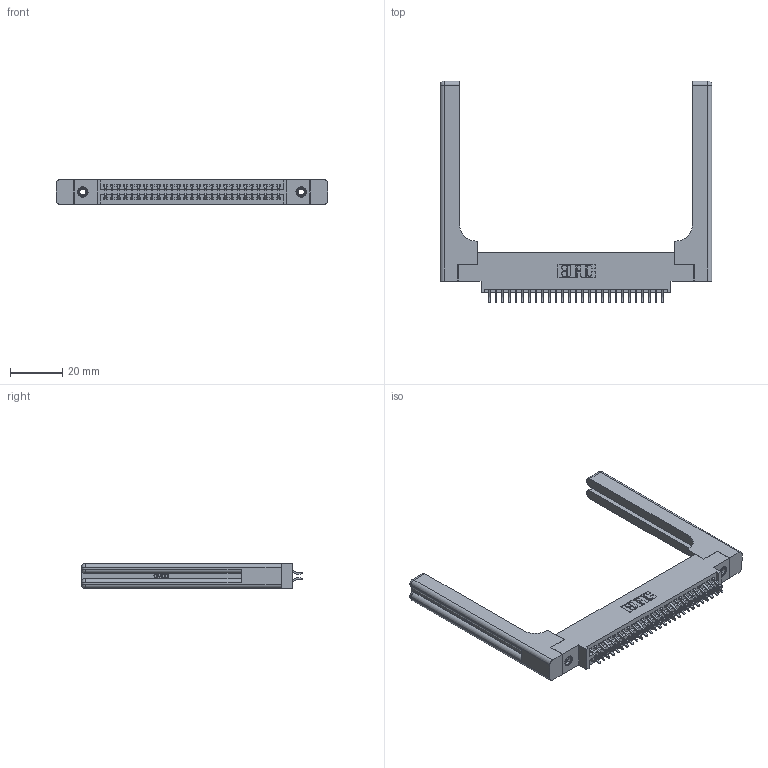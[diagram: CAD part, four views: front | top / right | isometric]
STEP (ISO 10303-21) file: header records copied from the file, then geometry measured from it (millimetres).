
FILE_DESCRIPTION (( 'STEP AP203' ), '1' );
FILE_NAME ('395-054-556-858.STEP', '2019-10-19T17:33:46', ( '' ), ( '' ), 'SwSTEP 2.0', 'SolidWorks 2016', '' );
FILE_SCHEMA (( 'CONFIG_CONTROL_DESIGN' ));
Length unit declared in the file: inch
Products named in the file (5): 345-220-058_345-220-058; 395-054-556-858; 345 Part_0.170 Offset - 0.156 Dia-TH; 345-292-001_556 Tail; 345-250-001_345-250-001-102
Assembly tree (59 placements, depth 2):
  395-054-556-858
    345 Part_0.170 Offset - 0.156 Dia-TH
    345-292-001_556 Tail  x54
    345-250-001_345-250-001-102  x2
    345-220-058_345-220-058  x2
Bounding box: 103.61 x 84.51 x 9.4 mm (x, y, z)
Volume: 18284.8 mm3; surface area: 19364.9 mm2
Topology: 59 solids, 59 shells, 3410 faces, 10037 edges, 6598 vertices
Faces by surface type: plane 2230, cylinder 1120, bspline 36, cone 12, sphere 8, torus 4
Entity records: 28738 total; most frequent: CARTESIAN_POINT 5841, ORIENTED_EDGE 4560, DIRECTION 4088, EDGE_CURVE 2280, VECTOR 1940, LINE 1940, VERTEX_POINT 1510, AXIS2_PLACEMENT_3D 1074
